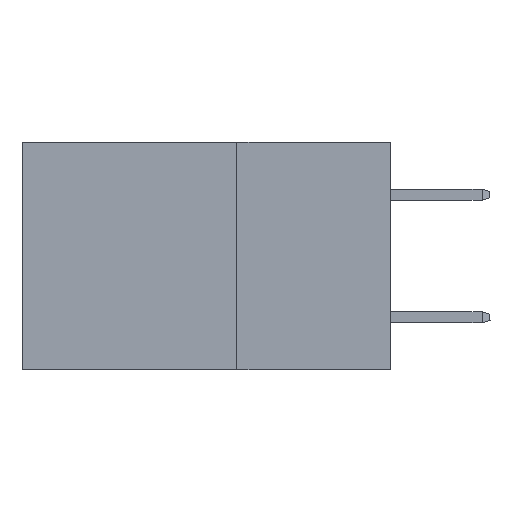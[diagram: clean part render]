
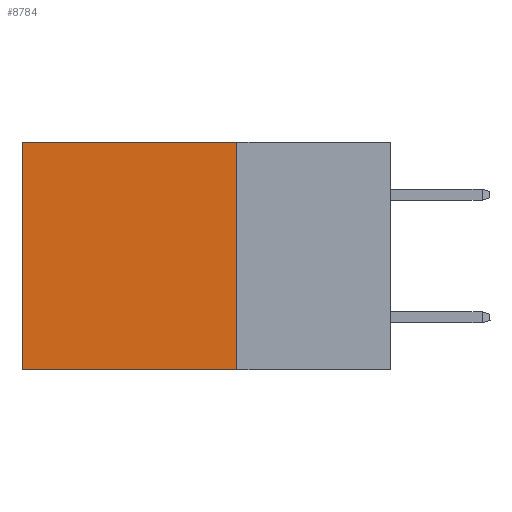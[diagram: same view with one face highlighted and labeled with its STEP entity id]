
A CAD part, left-side view. The second image highlights one B-rep face of the part: STEP entity #8784.
In plain terms, the highlighted planar face has unit normal (-1, 0, 0).
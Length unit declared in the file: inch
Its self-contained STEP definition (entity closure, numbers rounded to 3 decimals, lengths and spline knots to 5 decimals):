
#408 = ORIENTED_EDGE ( 'NONE', *, *, #1004, .F. ) ;
#803 = EDGE_CURVE ( 'NONE', #9375, #10554, #11477, .T. ) ;
#1004 = EDGE_CURVE ( 'NONE', #4922, #9375, #2705, .T. ) ;
#1146 = CARTESIAN_POINT ( 'NONE',  ( 0.2875, 0.6, -0.37 ) ) ;
#1216 = LINE ( 'NONE', #6553, #10895 ) ;
#1363 = DIRECTION ( 'NONE',  ( 0., 0., -1. ) ) ;
#1767 = CARTESIAN_POINT ( 'NONE',  ( 0.2875, 0.25, 0. ) ) ;
#1912 = VECTOR ( 'NONE', #8742, 39.37008 ) ;
#2466 = FACE_OUTER_BOUND ( 'NONE', #4240, .T. ) ;
#2705 = LINE ( 'NONE', #1767, #9805 ) ;
#3346 = CARTESIAN_POINT ( 'NONE',  ( 0.2875, 0.25, 0. ) ) ;
#3772 = VECTOR ( 'NONE', #11366, 39.37008 ) ;
#4049 = ORIENTED_EDGE ( 'NONE', *, *, #803, .F. ) ;
#4240 = EDGE_LOOP ( 'NONE', ( #6427, #4049, #408, #5864 ) ) ;
#4571 = EDGE_CURVE ( 'NONE', #8163, #10554, #6520, .T. ) ;
#4701 = DIRECTION ( 'NONE',  ( 0., 1., 0. ) ) ;
#4922 = VERTEX_POINT ( 'NONE', #7294 ) ;
#5226 = PLANE ( 'NONE',  #7340 ) ;
#5864 = ORIENTED_EDGE ( 'NONE', *, *, #7136, .T. ) ;
#6427 = ORIENTED_EDGE ( 'NONE', *, *, #4571, .T. ) ;
#6520 = LINE ( 'NONE', #8692, #3772 ) ;
#6553 = CARTESIAN_POINT ( 'NONE',  ( 0.2875, 0.25, 0. ) ) ;
#7073 = DIRECTION ( 'NONE',  ( 1., 0., 0. ) ) ;
#7136 = EDGE_CURVE ( 'NONE', #4922, #8163, #1216, .T. ) ;
#7294 = CARTESIAN_POINT ( 'NONE',  ( 0.2875, 0.25, 0. ) ) ;
#7340 = AXIS2_PLACEMENT_3D ( 'NONE', #3346, #7073, #1363 ) ;
#8022 = DIRECTION ( 'NONE',  ( 0., 0., -1. ) ) ;
#8163 = VERTEX_POINT ( 'NONE', #9702 ) ;
#8692 = CARTESIAN_POINT ( 'NONE',  ( 0.2875, 0.6, 0. ) ) ;
#8742 = DIRECTION ( 'NONE',  ( 0., 1., 0. ) ) ;
#8784 = ADVANCED_FACE ( 'NONE', ( #2466 ), #5226, .F. ) ;
#9375 = VERTEX_POINT ( 'NONE', #10653 ) ;
#9702 = CARTESIAN_POINT ( 'NONE',  ( 0.2875, 0.6, 0. ) ) ;
#9805 = VECTOR ( 'NONE', #8022, 39.37008 ) ;
#9941 = CARTESIAN_POINT ( 'NONE',  ( 0.2875, 0.25, -0.37 ) ) ;
#10554 = VERTEX_POINT ( 'NONE', #1146 ) ;
#10653 = CARTESIAN_POINT ( 'NONE',  ( 0.2875, 0.25, -0.37 ) ) ;
#10895 = VECTOR ( 'NONE', #4701, 39.37008 ) ;
#11366 = DIRECTION ( 'NONE',  ( 0., 0., -1. ) ) ;
#11477 = LINE ( 'NONE', #9941, #1912 ) ;
